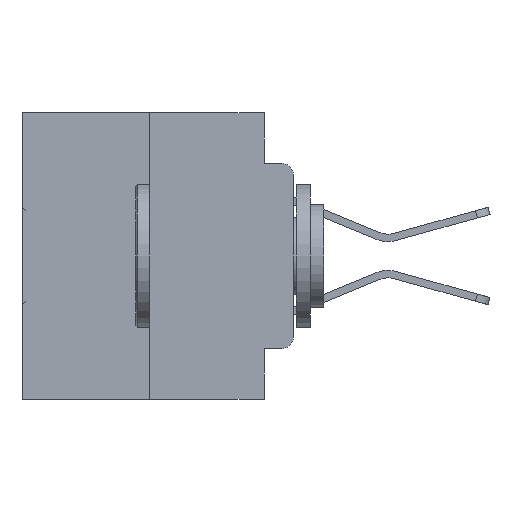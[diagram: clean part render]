
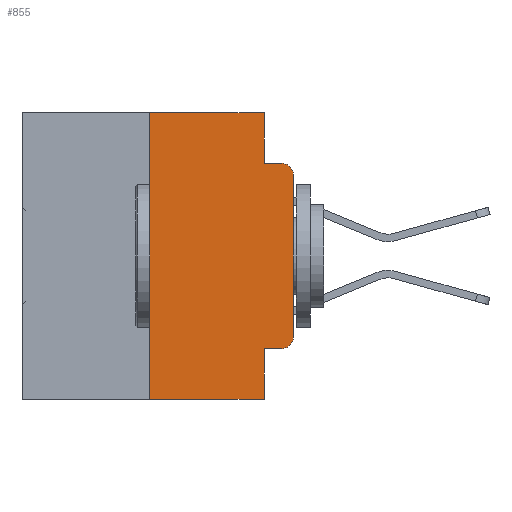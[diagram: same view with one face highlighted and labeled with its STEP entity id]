
A CAD part, left-side view. The second image highlights one B-rep face of the part: STEP entity #855.
In plain terms, the highlighted planar face has unit normal (-1, 0, 0).
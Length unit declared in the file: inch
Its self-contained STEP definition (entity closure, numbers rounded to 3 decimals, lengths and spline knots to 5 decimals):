
#11 = VERTEX_POINT ( 'NONE', #21134 ) ;
#193 = CARTESIAN_POINT ( 'NONE',  ( 0., 0.051, -0.5 ) ) ;
#201 = CIRCLE ( 'NONE', #4700, 0.02 ) ;
#221 = VECTOR ( 'NONE', #28647, 39.37008 ) ;
#290 = VECTOR ( 'NONE', #21664, 39.37008 ) ;
#855 = ADVANCED_FACE ( 'NONE', ( #1759 ), #14604, .F. ) ;
#943 = CARTESIAN_POINT ( 'NONE',  ( 0., 0.051, -0.0885 ) ) ;
#1759 = FACE_OUTER_BOUND ( 'NONE', #29287, .T. ) ;
#2013 = LINE ( 'NONE', #25907, #33655 ) ;
#2422 = DIRECTION ( 'NONE',  ( -1., 0., 0. ) ) ;
#2540 = DIRECTION ( 'NONE',  ( 0., 0., -1. ) ) ;
#2567 = CARTESIAN_POINT ( 'NONE',  ( 0., 0., 0. ) ) ;
#3138 = CARTESIAN_POINT ( 'NONE',  ( 0., 0.051, 0. ) ) ;
#3416 = CARTESIAN_POINT ( 'NONE',  ( 0., 0.25, 0. ) ) ;
#3457 = VERTEX_POINT ( 'NONE', #20468 ) ;
#3719 = AXIS2_PLACEMENT_3D ( 'NONE', #19088, #2422, #24202 ) ;
#3944 = VECTOR ( 'NONE', #14949, 39.37008 ) ;
#3977 = DIRECTION ( 'NONE',  ( -1., 0., 0. ) ) ;
#4700 = AXIS2_PLACEMENT_3D ( 'NONE', #17322, #3977, #26565 ) ;
#4752 = LINE ( 'NONE', #33724, #221 ) ;
#4970 = EDGE_CURVE ( 'NONE', #17501, #15920, #18892, .T. ) ;
#5096 = DIRECTION ( 'NONE',  ( 1., 0., 0. ) ) ;
#5277 = CARTESIAN_POINT ( 'NONE',  ( 0., 0.25, -0.5 ) ) ;
#5387 = ORIENTED_EDGE ( 'NONE', *, *, #5792, .F. ) ;
#5792 = EDGE_CURVE ( 'NONE', #15014, #7357, #30451, .T. ) ;
#7284 = ORIENTED_EDGE ( 'NONE', *, *, #14704, .T. ) ;
#7357 = VERTEX_POINT ( 'NONE', #3138 ) ;
#8355 = AXIS2_PLACEMENT_3D ( 'NONE', #25300, #5096, #25987 ) ;
#9384 = VECTOR ( 'NONE', #20058, 39.37008 ) ;
#9517 = LINE ( 'NONE', #31617, #3944 ) ;
#10341 = CARTESIAN_POINT ( 'NONE',  ( 0., 0., -0.1085 ) ) ;
#12176 = VERTEX_POINT ( 'NONE', #27058 ) ;
#12905 = ORIENTED_EDGE ( 'NONE', *, *, #16625, .F. ) ;
#13279 = CARTESIAN_POINT ( 'NONE',  ( 0., 0.473, -0.5 ) ) ;
#14604 = PLANE ( 'NONE',  #8355 ) ;
#14704 = EDGE_CURVE ( 'NONE', #18896, #15606, #23799, .T. ) ;
#14949 = DIRECTION ( 'NONE',  ( 0., 0., -1. ) ) ;
#15014 = VERTEX_POINT ( 'NONE', #19716 ) ;
#15606 = VERTEX_POINT ( 'NONE', #193 ) ;
#15724 = DIRECTION ( 'NONE',  ( 0., -1., 0. ) ) ;
#15920 = VERTEX_POINT ( 'NONE', #10341 ) ;
#16270 = DIRECTION ( 'NONE',  ( 0., 0., 1. ) ) ;
#16625 = EDGE_CURVE ( 'NONE', #18896, #15014, #26782, .T. ) ;
#17322 = CARTESIAN_POINT ( 'NONE',  ( 0., 0.02, -0.3915 ) ) ;
#17501 = VERTEX_POINT ( 'NONE', #29868 ) ;
#17603 = CARTESIAN_POINT ( 'NONE',  ( 0., 0.473, 0. ) ) ;
#18892 = LINE ( 'NONE', #2567, #22288 ) ;
#18896 = VERTEX_POINT ( 'NONE', #5277 ) ;
#19088 = CARTESIAN_POINT ( 'NONE',  ( 0., 0.02, -0.1085 ) ) ;
#19300 = EDGE_CURVE ( 'NONE', #15920, #3457, #22226, .T. ) ;
#19716 = CARTESIAN_POINT ( 'NONE',  ( 0., 0.25, 0. ) ) ;
#19721 = DIRECTION ( 'NONE',  ( 0., -1., 0. ) ) ;
#20058 = DIRECTION ( 'NONE',  ( 0., -1., 0. ) ) ;
#20373 = ORIENTED_EDGE ( 'NONE', *, *, #32449, .T. ) ;
#20468 = CARTESIAN_POINT ( 'NONE',  ( 0., 0.02, -0.0885 ) ) ;
#20788 = EDGE_CURVE ( 'NONE', #7357, #12176, #9517, .T. ) ;
#21134 = CARTESIAN_POINT ( 'NONE',  ( 0., 0.051, -0.4115 ) ) ;
#21169 = ORIENTED_EDGE ( 'NONE', *, *, #21198, .F. ) ;
#21198 = EDGE_CURVE ( 'NONE', #11, #15606, #2013, .T. ) ;
#21664 = DIRECTION ( 'NONE',  ( 0., 0., 1. ) ) ;
#21890 = ORIENTED_EDGE ( 'NONE', *, *, #19300, .T. ) ;
#22226 = CIRCLE ( 'NONE', #3719, 0.02 ) ;
#22288 = VECTOR ( 'NONE', #16270, 39.37008 ) ;
#23787 = ORIENTED_EDGE ( 'NONE', *, *, #4970, .T. ) ;
#23799 = LINE ( 'NONE', #13279, #24327 ) ;
#24202 = DIRECTION ( 'NONE',  ( 0., 0., -1. ) ) ;
#24327 = VECTOR ( 'NONE', #15724, 39.37008 ) ;
#25300 = CARTESIAN_POINT ( 'NONE',  ( 0., 0.473, 0. ) ) ;
#25528 = LINE ( 'NONE', #943, #25652 ) ;
#25652 = VECTOR ( 'NONE', #19721, 39.37008 ) ;
#25907 = CARTESIAN_POINT ( 'NONE',  ( 0., 0.051, 0. ) ) ;
#25987 = DIRECTION ( 'NONE',  ( 0., 0., -1. ) ) ;
#26256 = ORIENTED_EDGE ( 'NONE', *, *, #20788, .F. ) ;
#26565 = DIRECTION ( 'NONE',  ( 0., 0., -1. ) ) ;
#26782 = LINE ( 'NONE', #3416, #290 ) ;
#27058 = CARTESIAN_POINT ( 'NONE',  ( 0., 0.051, -0.0885 ) ) ;
#27218 = ORIENTED_EDGE ( 'NONE', *, *, #33020, .T. ) ;
#27941 = CARTESIAN_POINT ( 'NONE',  ( 0., 0.02, -0.4115 ) ) ;
#28647 = DIRECTION ( 'NONE',  ( 0., -1., 0. ) ) ;
#28790 = VERTEX_POINT ( 'NONE', #27941 ) ;
#29287 = EDGE_LOOP ( 'NONE', ( #23787, #21890, #30224, #26256, #5387, #12905, #7284, #21169, #27218, #20373 ) ) ;
#29868 = CARTESIAN_POINT ( 'NONE',  ( 0., 0., -0.3915 ) ) ;
#30224 = ORIENTED_EDGE ( 'NONE', *, *, #31320, .F. ) ;
#30451 = LINE ( 'NONE', #17603, #9384 ) ;
#31320 = EDGE_CURVE ( 'NONE', #12176, #3457, #25528, .T. ) ;
#31617 = CARTESIAN_POINT ( 'NONE',  ( 0., 0.051, 0. ) ) ;
#32449 = EDGE_CURVE ( 'NONE', #28790, #17501, #201, .T. ) ;
#33020 = EDGE_CURVE ( 'NONE', #11, #28790, #4752, .T. ) ;
#33655 = VECTOR ( 'NONE', #2540, 39.37008 ) ;
#33724 = CARTESIAN_POINT ( 'NONE',  ( 0., 0.051, -0.4115 ) ) ;
